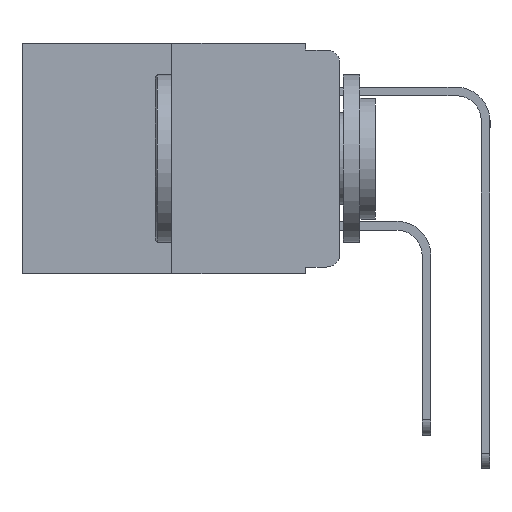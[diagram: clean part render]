
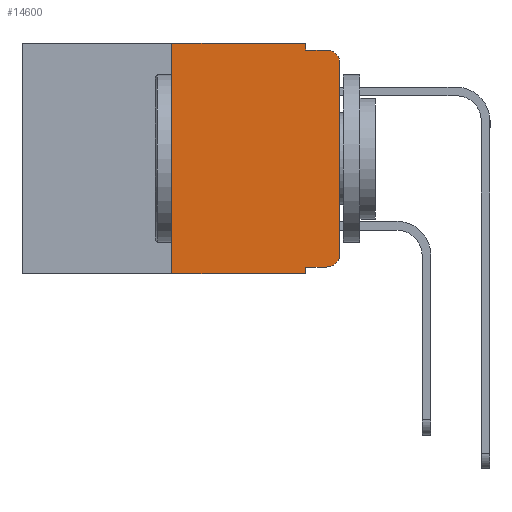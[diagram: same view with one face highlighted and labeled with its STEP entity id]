
A CAD part, left-side view. The second image highlights one B-rep face of the part: STEP entity #14600.
In plain terms, the highlighted planar face has unit normal (-1, 0, 0).
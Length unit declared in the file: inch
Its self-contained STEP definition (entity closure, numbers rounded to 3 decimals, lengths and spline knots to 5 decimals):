
#323 = VERTEX_POINT ( 'NONE', #10219 ) ;
#415 = AXIS2_PLACEMENT_3D ( 'NONE', #14149, #6197, #15408 ) ;
#678 = DIRECTION ( 'NONE',  ( 0., 0., 1. ) ) ;
#802 = EDGE_LOOP ( 'NONE', ( #6104, #7357, #3085, #3647, #3691, #3138, #3123, #3660, #3472, #3805 ) ) ;
#817 = EDGE_CURVE ( 'NONE', #323, #17018, #10717, .T. ) ;
#2047 = VERTEX_POINT ( 'NONE', #3968 ) ;
#2082 = CARTESIAN_POINT ( 'NONE',  ( 0., 0., 0. ) ) ;
#2293 = EDGE_CURVE ( 'NONE', #4455, #2047, #10469, .T. ) ;
#2440 = VERTEX_POINT ( 'NONE', #16139 ) ;
#2800 = PLANE ( 'NONE',  #14935 ) ;
#2985 = AXIS2_PLACEMENT_3D ( 'NONE', #5201, #14518, #6574 ) ;
#3085 = ORIENTED_EDGE ( 'NONE', *, *, #13573, .F. ) ;
#3123 = ORIENTED_EDGE ( 'NONE', *, *, #9924, .T. ) ;
#3138 = ORIENTED_EDGE ( 'NONE', *, *, #2293, .F. ) ;
#3394 = CARTESIAN_POINT ( 'NONE',  ( 0., 0.051, -0.01 ) ) ;
#3472 = ORIENTED_EDGE ( 'NONE', *, *, #5756, .T. ) ;
#3647 = ORIENTED_EDGE ( 'NONE', *, *, #4708, .F. ) ;
#3660 = ORIENTED_EDGE ( 'NONE', *, *, #817, .F. ) ;
#3691 = ORIENTED_EDGE ( 'NONE', *, *, #11730, .F. ) ;
#3805 = ORIENTED_EDGE ( 'NONE', *, *, #10606, .T. ) ;
#3822 = CARTESIAN_POINT ( 'NONE',  ( 0., 0., -0.03 ) ) ;
#3929 = VERTEX_POINT ( 'NONE', #12944 ) ;
#3968 = CARTESIAN_POINT ( 'NONE',  ( 0., 0.25, 0. ) ) ;
#4045 = VECTOR ( 'NONE', #8075, 39.37008 ) ;
#4187 = DIRECTION ( 'NONE',  ( 1., 0., 0. ) ) ;
#4455 = VERTEX_POINT ( 'NONE', #14644 ) ;
#4634 = DIRECTION ( 'NONE',  ( 0., 0., 1. ) ) ;
#4708 = EDGE_CURVE ( 'NONE', #13332, #9956, #14000, .T. ) ;
#4769 = LINE ( 'NONE', #7614, #11519 ) ;
#5201 = CARTESIAN_POINT ( 'NONE',  ( 0., 0.02, -0.03 ) ) ;
#5756 = EDGE_CURVE ( 'NONE', #323, #13523, #4769, .T. ) ;
#5921 = DIRECTION ( 'NONE',  ( 0., -1., 0. ) ) ;
#6007 = VECTOR ( 'NONE', #5921, 39.37008 ) ;
#6104 = ORIENTED_EDGE ( 'NONE', *, *, #15500, .T. ) ;
#6197 = DIRECTION ( 'NONE',  ( -1., 0., 0. ) ) ;
#6574 = DIRECTION ( 'NONE',  ( 0., 0., -1. ) ) ;
#6626 = CARTESIAN_POINT ( 'NONE',  ( 0., 0.25, 0. ) ) ;
#6642 = CARTESIAN_POINT ( 'NONE',  ( 0., 0.051, 0. ) ) ;
#6838 = DIRECTION ( 'NONE',  ( 0., 0., -1. ) ) ;
#7349 = CARTESIAN_POINT ( 'NONE',  ( 0., 0.051, 0. ) ) ;
#7357 = ORIENTED_EDGE ( 'NONE', *, *, #7556, .T. ) ;
#7384 = DIRECTION ( 'NONE',  ( 0., -1., 0. ) ) ;
#7556 = EDGE_CURVE ( 'NONE', #7572, #3929, #11457, .T. ) ;
#7572 = VERTEX_POINT ( 'NONE', #3822 ) ;
#7614 = CARTESIAN_POINT ( 'NONE',  ( 0., 0.051, -0.333 ) ) ;
#7655 = LINE ( 'NONE', #14668, #4045 ) ;
#7789 = LINE ( 'NONE', #2082, #10960 ) ;
#8075 = DIRECTION ( 'NONE',  ( 0., -1., 0. ) ) ;
#8670 = FACE_OUTER_BOUND ( 'NONE', #802, .T. ) ;
#8856 = CARTESIAN_POINT ( 'NONE',  ( 0., 0.051, 0. ) ) ;
#9648 = LINE ( 'NONE', #16574, #10061 ) ;
#9924 = EDGE_CURVE ( 'NONE', #4455, #17018, #9648, .T. ) ;
#9956 = VERTEX_POINT ( 'NONE', #3394 ) ;
#10061 = VECTOR ( 'NONE', #7384, 39.37008 ) ;
#10219 = CARTESIAN_POINT ( 'NONE',  ( 0., 0.051, -0.333 ) ) ;
#10253 = CIRCLE ( 'NONE', #415, 0.02 ) ;
#10469 = LINE ( 'NONE', #6626, #13145 ) ;
#10606 = EDGE_CURVE ( 'NONE', #13523, #2440, #10253, .T. ) ;
#10717 = LINE ( 'NONE', #6642, #17155 ) ;
#10960 = VECTOR ( 'NONE', #678, 39.37008 ) ;
#11457 = CIRCLE ( 'NONE', #2985, 0.02 ) ;
#11519 = VECTOR ( 'NONE', #16783, 39.37008 ) ;
#11730 = EDGE_CURVE ( 'NONE', #2047, #13332, #15709, .T. ) ;
#12196 = CARTESIAN_POINT ( 'NONE',  ( 0., 0.473, 0. ) ) ;
#12944 = CARTESIAN_POINT ( 'NONE',  ( 0., 0.02, -0.01 ) ) ;
#13145 = VECTOR ( 'NONE', #4634, 39.37008 ) ;
#13323 = CARTESIAN_POINT ( 'NONE',  ( 0., 0.02, -0.333 ) ) ;
#13332 = VERTEX_POINT ( 'NONE', #8856 ) ;
#13523 = VERTEX_POINT ( 'NONE', #13323 ) ;
#13529 = CARTESIAN_POINT ( 'NONE',  ( 0., 0.051, -0.343 ) ) ;
#13557 = DIRECTION ( 'NONE',  ( 0., 0., -1. ) ) ;
#13573 = EDGE_CURVE ( 'NONE', #9956, #3929, #7655, .T. ) ;
#13597 = VECTOR ( 'NONE', #15792, 39.37008 ) ;
#13902 = CARTESIAN_POINT ( 'NONE',  ( 0., 0.473, 0. ) ) ;
#14000 = LINE ( 'NONE', #7349, #13597 ) ;
#14149 = CARTESIAN_POINT ( 'NONE',  ( 0., 0.02, -0.313 ) ) ;
#14518 = DIRECTION ( 'NONE',  ( -1., 0., 0. ) ) ;
#14600 = ADVANCED_FACE ( 'NONE', ( #8670 ), #2800, .F. ) ;
#14644 = CARTESIAN_POINT ( 'NONE',  ( 0., 0.25, -0.343 ) ) ;
#14668 = CARTESIAN_POINT ( 'NONE',  ( 0., 0.051, -0.01 ) ) ;
#14935 = AXIS2_PLACEMENT_3D ( 'NONE', #12196, #4187, #13557 ) ;
#15408 = DIRECTION ( 'NONE',  ( 0., 0., -1. ) ) ;
#15500 = EDGE_CURVE ( 'NONE', #2440, #7572, #7789, .T. ) ;
#15709 = LINE ( 'NONE', #13902, #6007 ) ;
#15792 = DIRECTION ( 'NONE',  ( 0., 0., -1. ) ) ;
#16139 = CARTESIAN_POINT ( 'NONE',  ( 0., 0., -0.313 ) ) ;
#16574 = CARTESIAN_POINT ( 'NONE',  ( 0., 0.473, -0.343 ) ) ;
#16783 = DIRECTION ( 'NONE',  ( 0., -1., 0. ) ) ;
#17018 = VERTEX_POINT ( 'NONE', #13529 ) ;
#17155 = VECTOR ( 'NONE', #6838, 39.37008 ) ;
